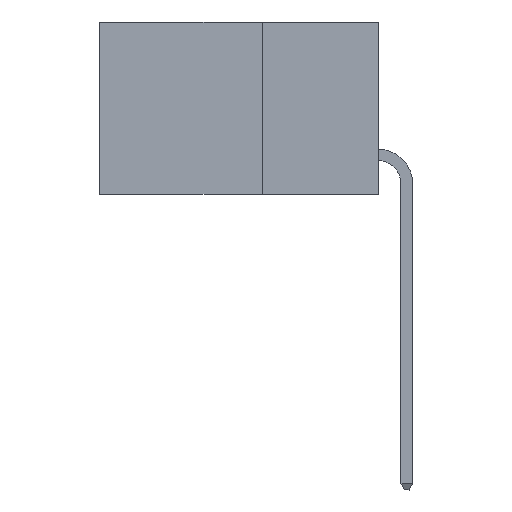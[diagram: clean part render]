
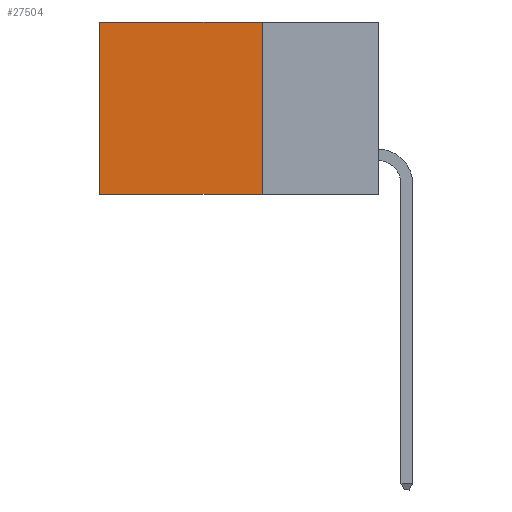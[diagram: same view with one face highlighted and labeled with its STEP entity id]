
A CAD part, left-side view. The second image highlights one B-rep face of the part: STEP entity #27504.
In plain terms, the highlighted planar face has unit normal (-1, 0, 0).
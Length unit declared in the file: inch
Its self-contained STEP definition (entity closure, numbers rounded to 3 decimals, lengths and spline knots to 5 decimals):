
#18 = VERTEX_POINT ( 'NONE', #24879 ) ;
#251 = VERTEX_POINT ( 'NONE', #19592 ) ;
#3149 = EDGE_CURVE ( 'NONE', #251, #20439, #11510, .T. ) ;
#3439 = DIRECTION ( 'NONE',  ( 0., 0., -1. ) ) ;
#4446 = EDGE_CURVE ( 'NONE', #18, #21768, #4721, .T. ) ;
#4721 = LINE ( 'NONE', #10145, #6239 ) ;
#5489 = CARTESIAN_POINT ( 'NONE',  ( 0.298, 0.6, 0. ) ) ;
#6046 = CARTESIAN_POINT ( 'NONE',  ( 0.298, 0.25, 0. ) ) ;
#6239 = VECTOR ( 'NONE', #19597, 39.37008 ) ;
#6477 = CARTESIAN_POINT ( 'NONE',  ( 0.298, 0.6, 0. ) ) ;
#6869 = EDGE_LOOP ( 'NONE', ( #26746, #28054, #7567, #20118 ) ) ;
#7567 = ORIENTED_EDGE ( 'NONE', *, *, #24433, .F. ) ;
#8426 = PLANE ( 'NONE',  #9536 ) ;
#9536 = AXIS2_PLACEMENT_3D ( 'NONE', #6046, #29544, #3439 ) ;
#9993 = CARTESIAN_POINT ( 'NONE',  ( 0.298, 0.6, -0.37 ) ) ;
#10145 = CARTESIAN_POINT ( 'NONE',  ( 0.298, 0.25, 0. ) ) ;
#10305 = CARTESIAN_POINT ( 'NONE',  ( 0.298, 0.25, 0. ) ) ;
#11510 = LINE ( 'NONE', #23614, #16312 ) ;
#12870 = VECTOR ( 'NONE', #13511, 39.37008 ) ;
#13511 = DIRECTION ( 'NONE',  ( 0., 0., -1. ) ) ;
#16182 = EDGE_CURVE ( 'NONE', #21768, #20439, #26968, .T. ) ;
#16312 = VECTOR ( 'NONE', #28589, 39.37008 ) ;
#19592 = CARTESIAN_POINT ( 'NONE',  ( 0.298, 0.25, -0.37 ) ) ;
#19597 = DIRECTION ( 'NONE',  ( 0., 1., 0. ) ) ;
#20118 = ORIENTED_EDGE ( 'NONE', *, *, #4446, .T. ) ;
#20439 = VERTEX_POINT ( 'NONE', #9993 ) ;
#21768 = VERTEX_POINT ( 'NONE', #5489 ) ;
#23433 = VECTOR ( 'NONE', #24097, 39.37008 ) ;
#23614 = CARTESIAN_POINT ( 'NONE',  ( 0.298, 0.25, -0.37 ) ) ;
#24097 = DIRECTION ( 'NONE',  ( 0., 0., -1. ) ) ;
#24433 = EDGE_CURVE ( 'NONE', #18, #251, #27896, .T. ) ;
#24879 = CARTESIAN_POINT ( 'NONE',  ( 0.298, 0.25, 0. ) ) ;
#25108 = FACE_OUTER_BOUND ( 'NONE', #6869, .T. ) ;
#26746 = ORIENTED_EDGE ( 'NONE', *, *, #16182, .T. ) ;
#26968 = LINE ( 'NONE', #6477, #12870 ) ;
#27504 = ADVANCED_FACE ( 'NONE', ( #25108 ), #8426, .F. ) ;
#27896 = LINE ( 'NONE', #10305, #23433 ) ;
#28054 = ORIENTED_EDGE ( 'NONE', *, *, #3149, .F. ) ;
#28589 = DIRECTION ( 'NONE',  ( 0., 1., 0. ) ) ;
#29544 = DIRECTION ( 'NONE',  ( 1., 0., 0. ) ) ;
